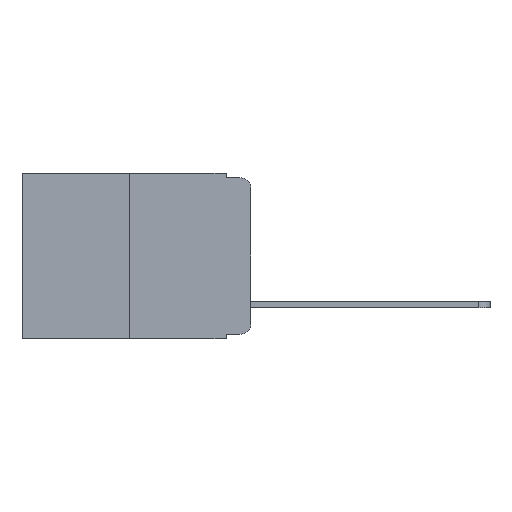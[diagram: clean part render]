
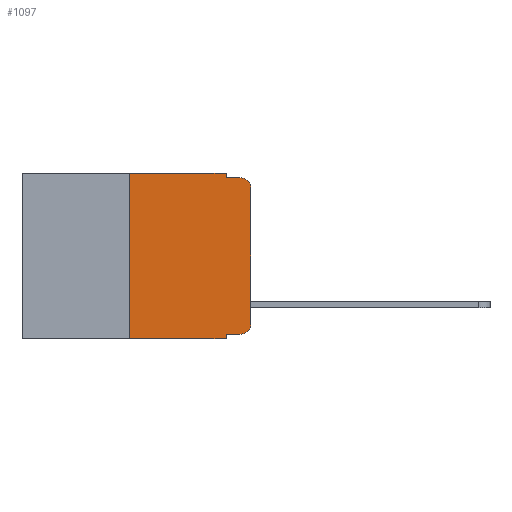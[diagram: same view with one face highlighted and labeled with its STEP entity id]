
A CAD part, left-side view. The second image highlights one B-rep face of the part: STEP entity #1097.
In plain terms, the highlighted planar face has unit normal (-1, 0, 0).
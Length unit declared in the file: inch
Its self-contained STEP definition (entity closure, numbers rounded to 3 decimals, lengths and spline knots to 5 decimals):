
#93 = LINE ( 'NONE', #7963, #16836 ) ;
#738 = VECTOR ( 'NONE', #6270, 39.37008 ) ;
#994 = DIRECTION ( 'NONE',  ( 0., 0., 1. ) ) ;
#1081 = VERTEX_POINT ( 'NONE', #16607 ) ;
#1097 = ADVANCED_FACE ( 'NONE', ( #17430 ), #13427, .F. ) ;
#1356 = LINE ( 'NONE', #16841, #738 ) ;
#2422 = VERTEX_POINT ( 'NONE', #13095 ) ;
#2801 = CARTESIAN_POINT ( 'NONE',  ( 0., 0.051, 0. ) ) ;
#2823 = VECTOR ( 'NONE', #5614, 39.37008 ) ;
#2893 = CARTESIAN_POINT ( 'NONE',  ( 0., 0.051, 0. ) ) ;
#3268 = CARTESIAN_POINT ( 'NONE',  ( 0., 0.02, -0.313 ) ) ;
#3441 = CARTESIAN_POINT ( 'NONE',  ( 0., 0.25, -0.343 ) ) ;
#3918 = VECTOR ( 'NONE', #17249, 39.37008 ) ;
#4027 = EDGE_LOOP ( 'NONE', ( #16067, #10030, #8144, #18112, #5635, #16168, #15655, #17053, #19925, #8479 ) ) ;
#4478 = VECTOR ( 'NONE', #994, 39.37008 ) ;
#4533 = CARTESIAN_POINT ( 'NONE',  ( 0., 0., -0.03 ) ) ;
#4595 = DIRECTION ( 'NONE',  ( -1., 0., 0. ) ) ;
#4986 = VERTEX_POINT ( 'NONE', #11530 ) ;
#5020 = LINE ( 'NONE', #2801, #9501 ) ;
#5059 = DIRECTION ( 'NONE',  ( 0., 0., -1. ) ) ;
#5069 = LINE ( 'NONE', #5860, #20022 ) ;
#5585 = CIRCLE ( 'NONE', #12447, 0.02 ) ;
#5614 = DIRECTION ( 'NONE',  ( 0., -1., 0. ) ) ;
#5635 = ORIENTED_EDGE ( 'NONE', *, *, #8509, .F. ) ;
#5860 = CARTESIAN_POINT ( 'NONE',  ( 0., 0.473, 0. ) ) ;
#6270 = DIRECTION ( 'NONE',  ( 0., 0., 1. ) ) ;
#6830 = CARTESIAN_POINT ( 'NONE',  ( 0., 0.051, -0.343 ) ) ;
#6947 = CARTESIAN_POINT ( 'NONE',  ( 0., 0., -0.313 ) ) ;
#7128 = VERTEX_POINT ( 'NONE', #4533 ) ;
#7455 = CARTESIAN_POINT ( 'NONE',  ( 0., 0.473, 0. ) ) ;
#7946 = VERTEX_POINT ( 'NONE', #19120 ) ;
#7963 = CARTESIAN_POINT ( 'NONE',  ( 0., 0.051, -0.01 ) ) ;
#8144 = ORIENTED_EDGE ( 'NONE', *, *, #9201, .F. ) ;
#8207 = DIRECTION ( 'NONE',  ( 0., 0., -1. ) ) ;
#8479 = ORIENTED_EDGE ( 'NONE', *, *, #9229, .T. ) ;
#8491 = LINE ( 'NONE', #2893, #3918 ) ;
#8509 = EDGE_CURVE ( 'NONE', #7946, #2422, #5069, .T. ) ;
#8915 = EDGE_CURVE ( 'NONE', #20289, #11191, #16852, .T. ) ;
#9172 = EDGE_CURVE ( 'NONE', #20308, #7128, #1356, .T. ) ;
#9199 = EDGE_CURVE ( 'NONE', #7128, #17862, #5585, .T. ) ;
#9201 = EDGE_CURVE ( 'NONE', #1081, #17862, #93, .T. ) ;
#9202 = EDGE_CURVE ( 'NONE', #2422, #1081, #5020, .T. ) ;
#9205 = EDGE_CURVE ( 'NONE', #20289, #7946, #13175, .T. ) ;
#9223 = EDGE_CURVE ( 'NONE', #4986, #11191, #8491, .T. ) ;
#9224 = EDGE_CURVE ( 'NONE', #4986, #12490, #17250, .T. ) ;
#9229 = EDGE_CURVE ( 'NONE', #12490, #20308, #19983, .T. ) ;
#9501 = VECTOR ( 'NONE', #9672, 39.37008 ) ;
#9672 = DIRECTION ( 'NONE',  ( 0., 0., -1. ) ) ;
#10026 = DIRECTION ( 'NONE',  ( 0., -1., 0. ) ) ;
#10030 = ORIENTED_EDGE ( 'NONE', *, *, #9199, .T. ) ;
#11191 = VERTEX_POINT ( 'NONE', #6830 ) ;
#11530 = CARTESIAN_POINT ( 'NONE',  ( 0., 0.051, -0.333 ) ) ;
#12447 = AXIS2_PLACEMENT_3D ( 'NONE', #14204, #4595, #15604 ) ;
#12490 = VERTEX_POINT ( 'NONE', #17064 ) ;
#12734 = VECTOR ( 'NONE', #10026, 39.37008 ) ;
#13095 = CARTESIAN_POINT ( 'NONE',  ( 0., 0.051, 0. ) ) ;
#13175 = LINE ( 'NONE', #19652, #4478 ) ;
#13400 = AXIS2_PLACEMENT_3D ( 'NONE', #3268, #14568, #5059 ) ;
#13427 = PLANE ( 'NONE',  #18733 ) ;
#13728 = DIRECTION ( 'NONE',  ( 1., 0., 0. ) ) ;
#14204 = CARTESIAN_POINT ( 'NONE',  ( 0., 0.02, -0.03 ) ) ;
#14568 = DIRECTION ( 'NONE',  ( -1., 0., 0. ) ) ;
#15006 = CARTESIAN_POINT ( 'NONE',  ( 0., 0.473, -0.343 ) ) ;
#15335 = CARTESIAN_POINT ( 'NONE',  ( 0., 0.02, -0.01 ) ) ;
#15604 = DIRECTION ( 'NONE',  ( 0., 0., -1. ) ) ;
#15655 = ORIENTED_EDGE ( 'NONE', *, *, #8915, .T. ) ;
#15902 = CARTESIAN_POINT ( 'NONE',  ( 0., 0.051, -0.333 ) ) ;
#16067 = ORIENTED_EDGE ( 'NONE', *, *, #9172, .T. ) ;
#16168 = ORIENTED_EDGE ( 'NONE', *, *, #9205, .F. ) ;
#16607 = CARTESIAN_POINT ( 'NONE',  ( 0., 0.051, -0.01 ) ) ;
#16836 = VECTOR ( 'NONE', #16958, 39.37008 ) ;
#16841 = CARTESIAN_POINT ( 'NONE',  ( 0., 0., 0. ) ) ;
#16852 = LINE ( 'NONE', #15006, #2823 ) ;
#16958 = DIRECTION ( 'NONE',  ( 0., -1., 0. ) ) ;
#17053 = ORIENTED_EDGE ( 'NONE', *, *, #9223, .F. ) ;
#17064 = CARTESIAN_POINT ( 'NONE',  ( 0., 0.02, -0.333 ) ) ;
#17249 = DIRECTION ( 'NONE',  ( 0., 0., -1. ) ) ;
#17250 = LINE ( 'NONE', #15902, #12734 ) ;
#17430 = FACE_OUTER_BOUND ( 'NONE', #4027, .T. ) ;
#17862 = VERTEX_POINT ( 'NONE', #15335 ) ;
#17902 = DIRECTION ( 'NONE',  ( 0., -1., 0. ) ) ;
#18112 = ORIENTED_EDGE ( 'NONE', *, *, #9202, .F. ) ;
#18733 = AXIS2_PLACEMENT_3D ( 'NONE', #7455, #13728, #8207 ) ;
#19120 = CARTESIAN_POINT ( 'NONE',  ( 0., 0.25, 0. ) ) ;
#19652 = CARTESIAN_POINT ( 'NONE',  ( 0., 0.25, 0. ) ) ;
#19925 = ORIENTED_EDGE ( 'NONE', *, *, #9224, .T. ) ;
#19983 = CIRCLE ( 'NONE', #13400, 0.02 ) ;
#20022 = VECTOR ( 'NONE', #17902, 39.37008 ) ;
#20289 = VERTEX_POINT ( 'NONE', #3441 ) ;
#20308 = VERTEX_POINT ( 'NONE', #6947 ) ;
